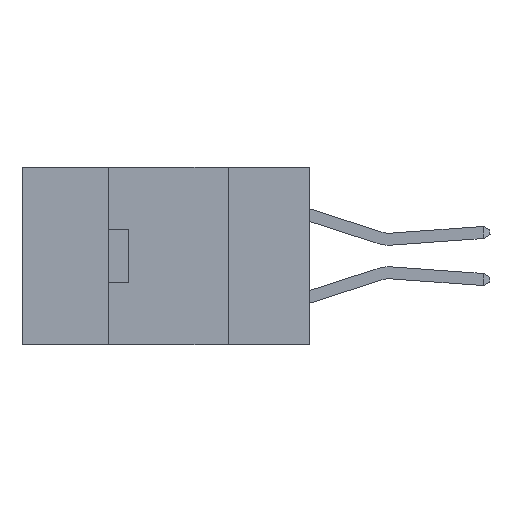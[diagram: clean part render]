
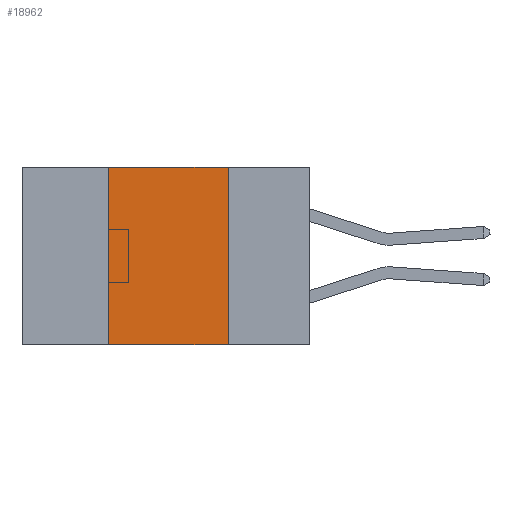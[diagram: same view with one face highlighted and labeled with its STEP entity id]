
A CAD part, left-side view. The second image highlights one B-rep face of the part: STEP entity #18962.
In plain terms, the highlighted planar face has unit normal (-1, 0, 0).
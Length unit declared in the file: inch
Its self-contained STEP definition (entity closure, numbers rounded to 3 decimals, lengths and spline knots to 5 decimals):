
#8 = CARTESIAN_POINT ( 'NONE',  ( 0., 0.42, -0.37 ) ) ;
#3710 = LINE ( 'NONE', #18985, #14056 ) ;
#4015 = DIRECTION ( 'NONE',  ( 0., -1., 0. ) ) ;
#5850 = LINE ( 'NONE', #18620, #16786 ) ;
#6781 = VERTEX_POINT ( 'NONE', #8 ) ;
#7904 = LINE ( 'NONE', #14097, #18187 ) ;
#8383 = ORIENTED_EDGE ( 'NONE', *, *, #21101, .T. ) ;
#9611 = CARTESIAN_POINT ( 'NONE',  ( 0., 0.6, 0. ) ) ;
#10270 = VERTEX_POINT ( 'NONE', #20499 ) ;
#11105 = VECTOR ( 'NONE', #4015, 39.37008 ) ;
#11576 = ORIENTED_EDGE ( 'NONE', *, *, #26418, .F. ) ;
#11682 = DIRECTION ( 'NONE',  ( 0., 0., -1. ) ) ;
#11755 = LINE ( 'NONE', #16343, #11105 ) ;
#13559 = AXIS2_PLACEMENT_3D ( 'NONE', #9611, #23994, #11682 ) ;
#14056 = VECTOR ( 'NONE', #21058, 39.37008 ) ;
#14097 = CARTESIAN_POINT ( 'NONE',  ( 0., 0.17, -0.37 ) ) ;
#14507 = DIRECTION ( 'NONE',  ( 0., 0., 1. ) ) ;
#16127 = DIRECTION ( 'NONE',  ( 0., 0., -1. ) ) ;
#16343 = CARTESIAN_POINT ( 'NONE',  ( 0., 0.6, -0.37 ) ) ;
#16727 = ORIENTED_EDGE ( 'NONE', *, *, #22998, .F. ) ;
#16786 = VECTOR ( 'NONE', #14507, 39.37008 ) ;
#18187 = VECTOR ( 'NONE', #16127, 39.37008 ) ;
#18620 = CARTESIAN_POINT ( 'NONE',  ( 0., 0.42, -0.37 ) ) ;
#18697 = EDGE_CURVE ( 'NONE', #10270, #19909, #3710, .T. ) ;
#18962 = ADVANCED_FACE ( 'NONE', ( #19179 ), #21948, .F. ) ;
#18982 = VERTEX_POINT ( 'NONE', #19990 ) ;
#18985 = CARTESIAN_POINT ( 'NONE',  ( 0., 0.6, 0. ) ) ;
#19179 = FACE_OUTER_BOUND ( 'NONE', #26196, .T. ) ;
#19909 = VERTEX_POINT ( 'NONE', #24315 ) ;
#19990 = CARTESIAN_POINT ( 'NONE',  ( 0., 0.17, -0.37 ) ) ;
#20499 = CARTESIAN_POINT ( 'NONE',  ( 0., 0.42, 0. ) ) ;
#21058 = DIRECTION ( 'NONE',  ( 0., -1., 0. ) ) ;
#21101 = EDGE_CURVE ( 'NONE', #6781, #18982, #11755, .T. ) ;
#21948 = PLANE ( 'NONE',  #13559 ) ;
#22998 = EDGE_CURVE ( 'NONE', #6781, #10270, #5850, .T. ) ;
#23994 = DIRECTION ( 'NONE',  ( 1., 0., 0. ) ) ;
#24315 = CARTESIAN_POINT ( 'NONE',  ( 0., 0.17, 0. ) ) ;
#25075 = ORIENTED_EDGE ( 'NONE', *, *, #18697, .F. ) ;
#26196 = EDGE_LOOP ( 'NONE', ( #11576, #25075, #16727, #8383 ) ) ;
#26418 = EDGE_CURVE ( 'NONE', #19909, #18982, #7904, .T. ) ;
